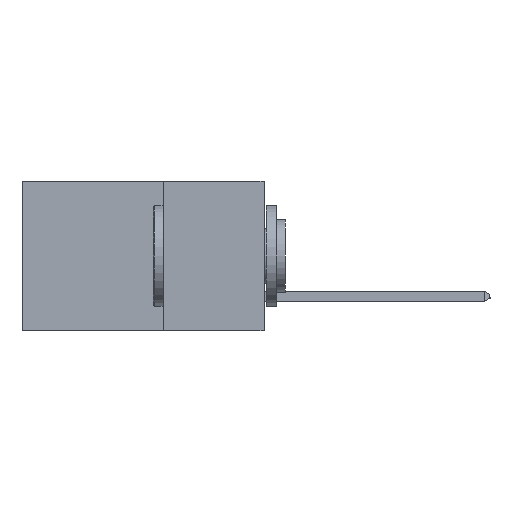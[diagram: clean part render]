
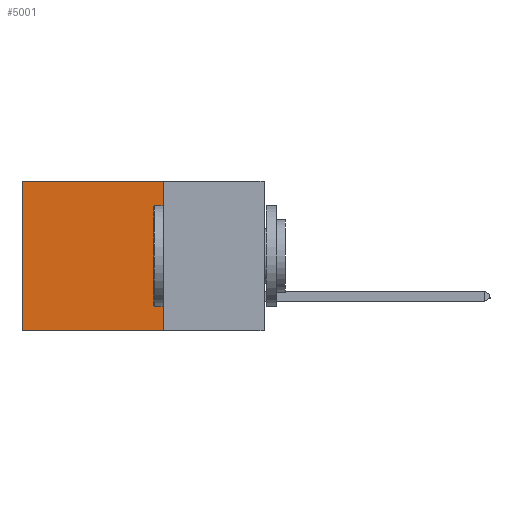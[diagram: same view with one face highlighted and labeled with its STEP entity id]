
A CAD part, left-side view. The second image highlights one B-rep face of the part: STEP entity #5001.
In plain terms, the highlighted planar face has unit normal (-1, 0, 0).
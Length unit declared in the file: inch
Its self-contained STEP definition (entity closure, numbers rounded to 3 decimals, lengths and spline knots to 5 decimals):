
#278 = VERTEX_POINT ( 'NONE', #8166 ) ;
#365 = VECTOR ( 'NONE', #9722, 39.37008 ) ;
#1608 = CARTESIAN_POINT ( 'NONE',  ( 0.298, 0.25, 0. ) ) ;
#1722 = ORIENTED_EDGE ( 'NONE', *, *, #9946, .T. ) ;
#2150 = FACE_OUTER_BOUND ( 'NONE', #5093, .T. ) ;
#2308 = VECTOR ( 'NONE', #3276, 39.37008 ) ;
#2623 = LINE ( 'NONE', #11178, #2308 ) ;
#2867 = ORIENTED_EDGE ( 'NONE', *, *, #11176, .F. ) ;
#2973 = LINE ( 'NONE', #1608, #365 ) ;
#3072 = EDGE_CURVE ( 'NONE', #6954, #8150, #4474, .T. ) ;
#3276 = DIRECTION ( 'NONE',  ( 0., 1., 0. ) ) ;
#3445 = PLANE ( 'NONE',  #5163 ) ;
#3823 = ORIENTED_EDGE ( 'NONE', *, *, #3072, .T. ) ;
#4474 = LINE ( 'NONE', #11298, #10930 ) ;
#4635 = VERTEX_POINT ( 'NONE', #10321 ) ;
#4696 = CARTESIAN_POINT ( 'NONE',  ( 0.298, 0.25, 0. ) ) ;
#4748 = DIRECTION ( 'NONE',  ( 0., 0., -1. ) ) ;
#4753 = DIRECTION ( 'NONE',  ( 1., 0., 0. ) ) ;
#5001 = ADVANCED_FACE ( 'NONE', ( #2150 ), #3445, .F. ) ;
#5093 = EDGE_LOOP ( 'NONE', ( #1722, #7671, #2867, #3823 ) ) ;
#5163 = AXIS2_PLACEMENT_3D ( 'NONE', #4696, #4753, #4748 ) ;
#5236 = VECTOR ( 'NONE', #8044, 39.37008 ) ;
#5799 = LINE ( 'NONE', #7139, #5236 ) ;
#6954 = VERTEX_POINT ( 'NONE', #9151 ) ;
#7139 = CARTESIAN_POINT ( 'NONE',  ( 0.298, 0.6, 0. ) ) ;
#7364 = CARTESIAN_POINT ( 'NONE',  ( 0.298, 0.6, 0. ) ) ;
#7671 = ORIENTED_EDGE ( 'NONE', *, *, #7903, .F. ) ;
#7903 = EDGE_CURVE ( 'NONE', #278, #4635, #2623, .T. ) ;
#8004 = DIRECTION ( 'NONE',  ( 0., 1., 0. ) ) ;
#8044 = DIRECTION ( 'NONE',  ( 0., 0., -1. ) ) ;
#8150 = VERTEX_POINT ( 'NONE', #7364 ) ;
#8166 = CARTESIAN_POINT ( 'NONE',  ( 0.298, 0.25, -0.37 ) ) ;
#9151 = CARTESIAN_POINT ( 'NONE',  ( 0.298, 0.25, 0. ) ) ;
#9722 = DIRECTION ( 'NONE',  ( 0., 0., -1. ) ) ;
#9946 = EDGE_CURVE ( 'NONE', #8150, #4635, #5799, .T. ) ;
#10321 = CARTESIAN_POINT ( 'NONE',  ( 0.298, 0.6, -0.37 ) ) ;
#10930 = VECTOR ( 'NONE', #8004, 39.37008 ) ;
#11176 = EDGE_CURVE ( 'NONE', #6954, #278, #2973, .T. ) ;
#11178 = CARTESIAN_POINT ( 'NONE',  ( 0.298, 0.25, -0.37 ) ) ;
#11298 = CARTESIAN_POINT ( 'NONE',  ( 0.298, 0.25, 0. ) ) ;
